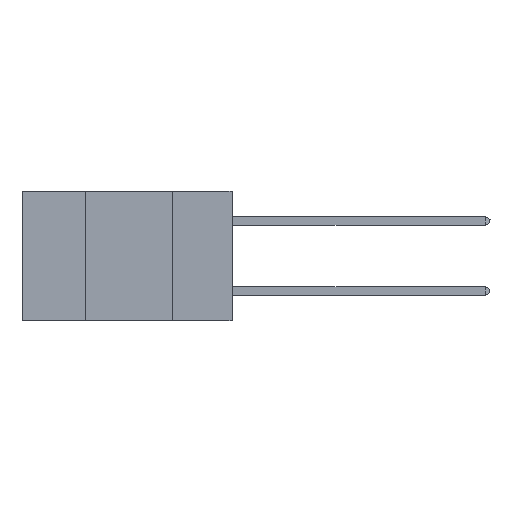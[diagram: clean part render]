
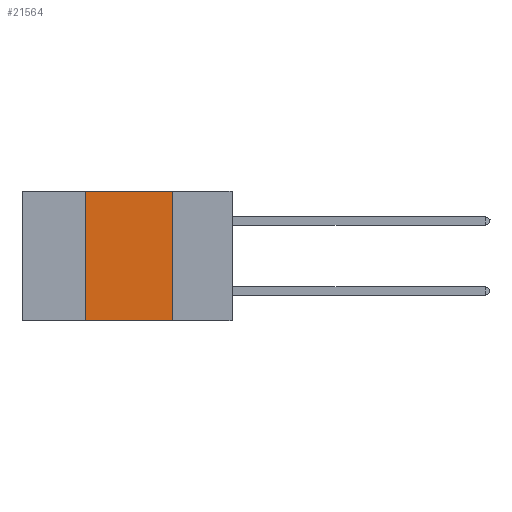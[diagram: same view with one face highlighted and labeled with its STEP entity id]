
A CAD part, left-side view. The second image highlights one B-rep face of the part: STEP entity #21564.
In plain terms, the highlighted planar face has unit normal (-1, 0, 0).
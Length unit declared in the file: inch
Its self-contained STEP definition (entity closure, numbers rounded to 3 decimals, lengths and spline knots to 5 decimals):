
#521 = CARTESIAN_POINT ( 'NONE',  ( 0., 0.17, 0. ) ) ;
#807 = VECTOR ( 'NONE', #22865, 39.37008 ) ;
#1353 = ORIENTED_EDGE ( 'NONE', *, *, #29600, .F. ) ;
#3194 = CARTESIAN_POINT ( 'NONE',  ( 0., 0.42, 0. ) ) ;
#3930 = VECTOR ( 'NONE', #15294, 39.37008 ) ;
#4082 = VERTEX_POINT ( 'NONE', #14306 ) ;
#4273 = CARTESIAN_POINT ( 'NONE',  ( 0., 0.42, -0.37 ) ) ;
#4767 = LINE ( 'NONE', #28947, #14582 ) ;
#5203 = EDGE_CURVE ( 'NONE', #17465, #5329, #23558, .T. ) ;
#5329 = VERTEX_POINT ( 'NONE', #521 ) ;
#5514 = ORIENTED_EDGE ( 'NONE', *, *, #31831, .F. ) ;
#5792 = LINE ( 'NONE', #3194, #3930 ) ;
#6904 = FACE_OUTER_BOUND ( 'NONE', #26192, .T. ) ;
#7803 = CARTESIAN_POINT ( 'NONE',  ( 0., 0.6, -0.37 ) ) ;
#10659 = DIRECTION ( 'NONE',  ( 0., 0., -1. ) ) ;
#13970 = EDGE_CURVE ( 'NONE', #25320, #4082, #22465, .T. ) ;
#14306 = CARTESIAN_POINT ( 'NONE',  ( 0., 0.17, -0.37 ) ) ;
#14582 = VECTOR ( 'NONE', #31743, 39.37008 ) ;
#15294 = DIRECTION ( 'NONE',  ( 0., 0., 1. ) ) ;
#15620 = PLANE ( 'NONE',  #34510 ) ;
#15832 = CARTESIAN_POINT ( 'NONE',  ( 0., 0.42, 0. ) ) ;
#17465 = VERTEX_POINT ( 'NONE', #15832 ) ;
#17594 = CARTESIAN_POINT ( 'NONE',  ( 0., 0.6, 0. ) ) ;
#21564 = ADVANCED_FACE ( 'NONE', ( #6904 ), #15620, .F. ) ;
#21961 = CARTESIAN_POINT ( 'NONE',  ( 0., 0.6, 0. ) ) ;
#22391 = ORIENTED_EDGE ( 'NONE', *, *, #5203, .F. ) ;
#22465 = LINE ( 'NONE', #7803, #807 ) ;
#22865 = DIRECTION ( 'NONE',  ( 0., -1., 0. ) ) ;
#23558 = LINE ( 'NONE', #17594, #31086 ) ;
#25320 = VERTEX_POINT ( 'NONE', #4273 ) ;
#26192 = EDGE_LOOP ( 'NONE', ( #1353, #22391, #5514, #32881 ) ) ;
#26536 = DIRECTION ( 'NONE',  ( 0., -1., 0. ) ) ;
#28947 = CARTESIAN_POINT ( 'NONE',  ( 0., 0.17, 0. ) ) ;
#29600 = EDGE_CURVE ( 'NONE', #5329, #4082, #4767, .T. ) ;
#31086 = VECTOR ( 'NONE', #26536, 39.37008 ) ;
#31097 = DIRECTION ( 'NONE',  ( 1., 0., 0. ) ) ;
#31743 = DIRECTION ( 'NONE',  ( 0., 0., -1. ) ) ;
#31831 = EDGE_CURVE ( 'NONE', #25320, #17465, #5792, .T. ) ;
#32881 = ORIENTED_EDGE ( 'NONE', *, *, #13970, .T. ) ;
#34510 = AXIS2_PLACEMENT_3D ( 'NONE', #21961, #31097, #10659 ) ;
